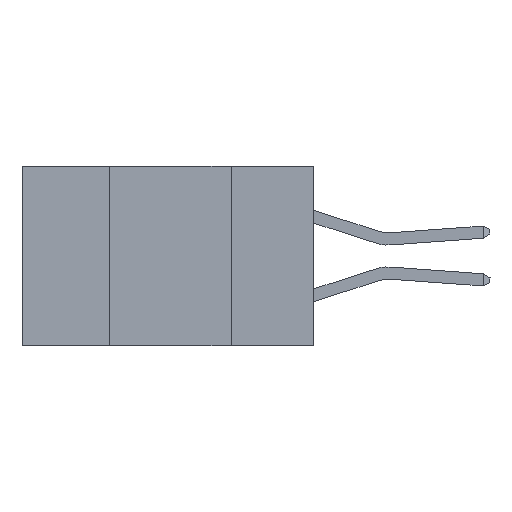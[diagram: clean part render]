
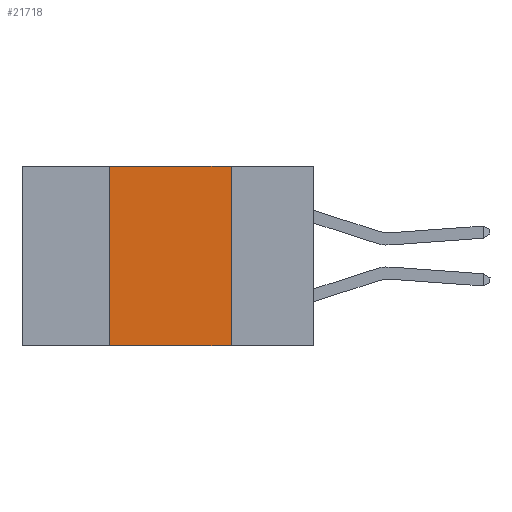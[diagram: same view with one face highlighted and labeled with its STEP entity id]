
A CAD part, left-side view. The second image highlights one B-rep face of the part: STEP entity #21718.
In plain terms, the highlighted planar face has unit normal (-1, 0, 0).
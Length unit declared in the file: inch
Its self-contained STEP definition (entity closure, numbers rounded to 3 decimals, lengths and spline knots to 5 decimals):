
#1751 = VERTEX_POINT ( 'NONE', #11669 ) ;
#2127 = FACE_OUTER_BOUND ( 'NONE', #26684, .T. ) ;
#3334 = EDGE_CURVE ( 'NONE', #12474, #26997, #13282, .T. ) ;
#4434 = ORIENTED_EDGE ( 'NONE', *, *, #18690, .F. ) ;
#5305 = PLANE ( 'NONE',  #26382 ) ;
#6271 = VERTEX_POINT ( 'NONE', #7586 ) ;
#6757 = ORIENTED_EDGE ( 'NONE', *, *, #21851, .F. ) ;
#7368 = CARTESIAN_POINT ( 'NONE',  ( 0., 0.6, 0. ) ) ;
#7423 = CARTESIAN_POINT ( 'NONE',  ( 0., 0.17, 0. ) ) ;
#7586 = CARTESIAN_POINT ( 'NONE',  ( 0., 0.42, -0.37 ) ) ;
#9247 = EDGE_CURVE ( 'NONE', #6271, #1751, #12511, .T. ) ;
#9537 = ORIENTED_EDGE ( 'NONE', *, *, #3334, .F. ) ;
#10215 = DIRECTION ( 'NONE',  ( 0., 0., 1. ) ) ;
#11669 = CARTESIAN_POINT ( 'NONE',  ( 0., 0.17, -0.37 ) ) ;
#12474 = VERTEX_POINT ( 'NONE', #14391 ) ;
#12511 = LINE ( 'NONE', #25026, #22673 ) ;
#13282 = LINE ( 'NONE', #14756, #17653 ) ;
#14391 = CARTESIAN_POINT ( 'NONE',  ( 0., 0.42, 0. ) ) ;
#14756 = CARTESIAN_POINT ( 'NONE',  ( 0., 0.6, 0. ) ) ;
#15005 = VECTOR ( 'NONE', #25648, 39.37008 ) ;
#15897 = ORIENTED_EDGE ( 'NONE', *, *, #9247, .T. ) ;
#16034 = DIRECTION ( 'NONE',  ( 0., -1., 0. ) ) ;
#16624 = CARTESIAN_POINT ( 'NONE',  ( 0., 0.42, 0. ) ) ;
#17653 = VECTOR ( 'NONE', #25560, 39.37008 ) ;
#18690 = EDGE_CURVE ( 'NONE', #26997, #1751, #21125, .T. ) ;
#21016 = VECTOR ( 'NONE', #10215, 39.37008 ) ;
#21125 = LINE ( 'NONE', #23740, #15005 ) ;
#21718 = ADVANCED_FACE ( 'NONE', ( #2127 ), #5305, .F. ) ;
#21851 = EDGE_CURVE ( 'NONE', #6271, #12474, #22381, .T. ) ;
#22381 = LINE ( 'NONE', #16624, #21016 ) ;
#22394 = DIRECTION ( 'NONE',  ( 1., 0., 0. ) ) ;
#22673 = VECTOR ( 'NONE', #16034, 39.37008 ) ;
#23740 = CARTESIAN_POINT ( 'NONE',  ( 0., 0.17, 0. ) ) ;
#25026 = CARTESIAN_POINT ( 'NONE',  ( 0., 0.6, -0.37 ) ) ;
#25560 = DIRECTION ( 'NONE',  ( 0., -1., 0. ) ) ;
#25648 = DIRECTION ( 'NONE',  ( 0., 0., -1. ) ) ;
#26382 = AXIS2_PLACEMENT_3D ( 'NONE', #7368, #22394, #26859 ) ;
#26684 = EDGE_LOOP ( 'NONE', ( #4434, #9537, #6757, #15897 ) ) ;
#26859 = DIRECTION ( 'NONE',  ( 0., 0., -1. ) ) ;
#26997 = VERTEX_POINT ( 'NONE', #7423 ) ;
